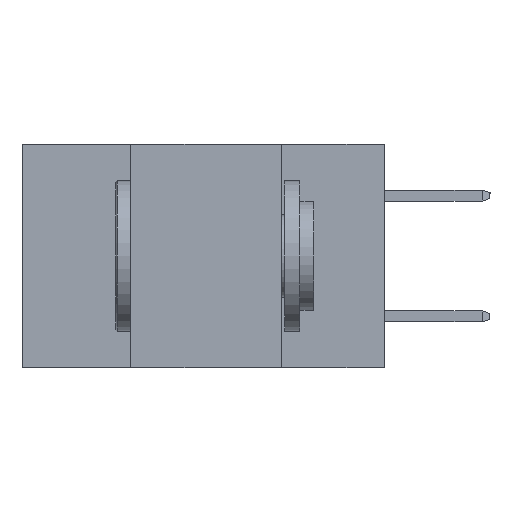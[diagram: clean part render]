
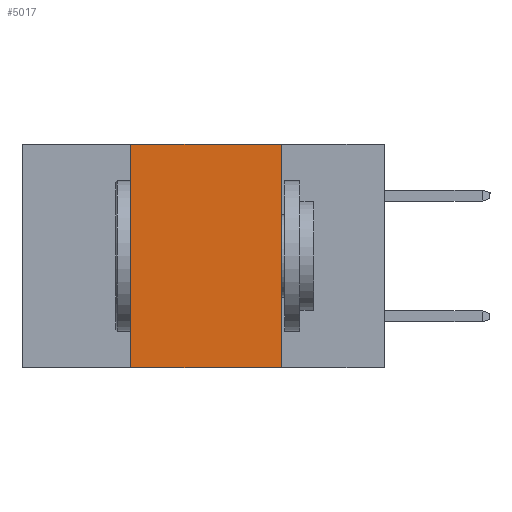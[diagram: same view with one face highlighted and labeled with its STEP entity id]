
A CAD part, left-side view. The second image highlights one B-rep face of the part: STEP entity #5017.
In plain terms, the highlighted planar face has unit normal (-1, 0, 0).
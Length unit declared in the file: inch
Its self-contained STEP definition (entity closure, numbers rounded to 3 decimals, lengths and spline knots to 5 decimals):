
#296 = VERTEX_POINT ( 'NONE', #7254 ) ;
#745 = ORIENTED_EDGE ( 'NONE', *, *, #3711, .F. ) ;
#1472 = ORIENTED_EDGE ( 'NONE', *, *, #4458, .F. ) ;
#1617 = VERTEX_POINT ( 'NONE', #1825 ) ;
#1825 = CARTESIAN_POINT ( 'NONE',  ( 0., 0.17, 0. ) ) ;
#2364 = EDGE_CURVE ( 'NONE', #12285, #9407, #8747, .T. ) ;
#2663 = VECTOR ( 'NONE', #10619, 39.37008 ) ;
#2888 = DIRECTION ( 'NONE',  ( 0., -1., 0. ) ) ;
#2895 = LINE ( 'NONE', #6753, #2663 ) ;
#3711 = EDGE_CURVE ( 'NONE', #296, #1617, #11448, .T. ) ;
#3941 = VECTOR ( 'NONE', #8939, 39.37008 ) ;
#3959 = CARTESIAN_POINT ( 'NONE',  ( 0., 0.6, -0.37 ) ) ;
#4458 = EDGE_CURVE ( 'NONE', #1617, #9407, #8353, .T. ) ;
#5017 = ADVANCED_FACE ( 'NONE', ( #8157 ), #8360, .F. ) ;
#5493 = DIRECTION ( 'NONE',  ( 0., 0., -1. ) ) ;
#6614 = ORIENTED_EDGE ( 'NONE', *, *, #9473, .F. ) ;
#6618 = CARTESIAN_POINT ( 'NONE',  ( 0., 0.6, 0. ) ) ;
#6753 = CARTESIAN_POINT ( 'NONE',  ( 0., 0.42, -0.37 ) ) ;
#7254 = CARTESIAN_POINT ( 'NONE',  ( 0., 0.42, 0. ) ) ;
#7407 = CARTESIAN_POINT ( 'NONE',  ( 0., 0.17, -0.37 ) ) ;
#7413 = DIRECTION ( 'NONE',  ( 1., 0., 0. ) ) ;
#7508 = EDGE_LOOP ( 'NONE', ( #1472, #745, #6614, #11179 ) ) ;
#8079 = VECTOR ( 'NONE', #2888, 39.37008 ) ;
#8157 = FACE_OUTER_BOUND ( 'NONE', #7508, .T. ) ;
#8353 = LINE ( 'NONE', #7407, #9126 ) ;
#8360 = PLANE ( 'NONE',  #9701 ) ;
#8747 = LINE ( 'NONE', #3959, #3941 ) ;
#8939 = DIRECTION ( 'NONE',  ( 0., -1., 0. ) ) ;
#9126 = VECTOR ( 'NONE', #5493, 39.37008 ) ;
#9407 = VERTEX_POINT ( 'NONE', #12220 ) ;
#9473 = EDGE_CURVE ( 'NONE', #12285, #296, #2895, .T. ) ;
#9701 = AXIS2_PLACEMENT_3D ( 'NONE', #12049, #7413, #12107 ) ;
#10619 = DIRECTION ( 'NONE',  ( 0., 0., 1. ) ) ;
#11179 = ORIENTED_EDGE ( 'NONE', *, *, #2364, .T. ) ;
#11448 = LINE ( 'NONE', #6618, #8079 ) ;
#11832 = CARTESIAN_POINT ( 'NONE',  ( 0., 0.42, -0.37 ) ) ;
#12049 = CARTESIAN_POINT ( 'NONE',  ( 0., 0.6, 0. ) ) ;
#12107 = DIRECTION ( 'NONE',  ( 0., 0., -1. ) ) ;
#12220 = CARTESIAN_POINT ( 'NONE',  ( 0., 0.17, -0.37 ) ) ;
#12285 = VERTEX_POINT ( 'NONE', #11832 ) ;
